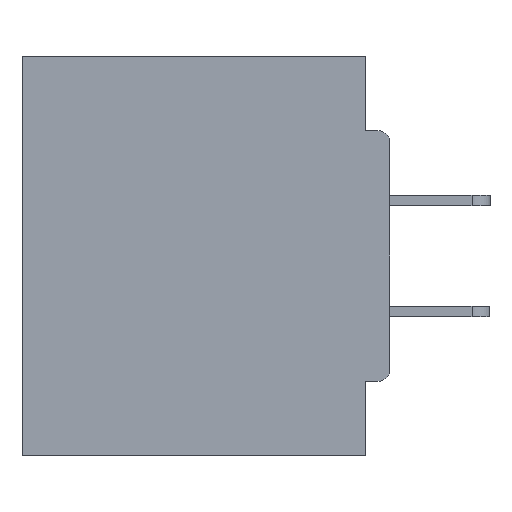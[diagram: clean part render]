
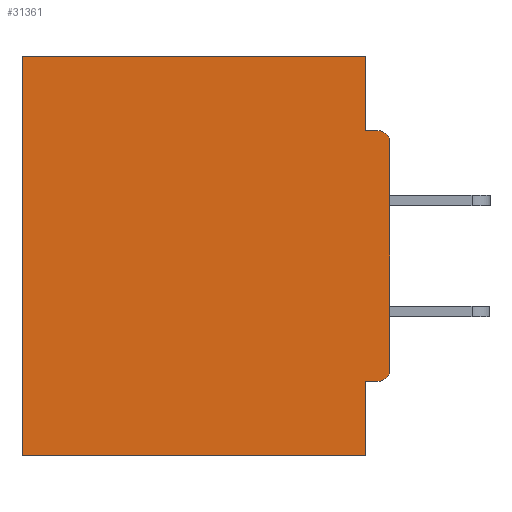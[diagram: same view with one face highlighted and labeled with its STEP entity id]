
A CAD part, left-side view. The second image highlights one B-rep face of the part: STEP entity #31361.
In plain terms, the highlighted planar face has unit normal (-1, 0, 0).
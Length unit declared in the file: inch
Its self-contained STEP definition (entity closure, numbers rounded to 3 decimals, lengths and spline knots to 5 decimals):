
#343 = VERTEX_POINT ( 'NONE', #32561 ) ;
#401 = VERTEX_POINT ( 'NONE', #16151 ) ;
#1222 = FACE_OUTER_BOUND ( 'NONE', #25110, .T. ) ;
#2314 = DIRECTION ( 'NONE',  ( 1., 0., 0. ) ) ;
#2408 = EDGE_CURVE ( 'NONE', #2842, #25228, #22369, .T. ) ;
#2842 = VERTEX_POINT ( 'NONE', #25498 ) ;
#3152 = DIRECTION ( 'NONE',  ( 0., 0., -1. ) ) ;
#3388 = ORIENTED_EDGE ( 'NONE', *, *, #12631, .T. ) ;
#3606 = CARTESIAN_POINT ( 'NONE',  ( 0.298, 0.015, -0.3915 ) ) ;
#3746 = ORIENTED_EDGE ( 'NONE', *, *, #28068, .F. ) ;
#3950 = VECTOR ( 'NONE', #13686, 39.37008 ) ;
#4068 = CARTESIAN_POINT ( 'NONE',  ( 0.298, 0., -0.0935 ) ) ;
#4237 = ORIENTED_EDGE ( 'NONE', *, *, #26782, .F. ) ;
#4886 = CARTESIAN_POINT ( 'NONE',  ( 0.298, 0., 0. ) ) ;
#5435 = DIRECTION ( 'NONE',  ( 0., 0., -1. ) ) ;
#5617 = DIRECTION ( 'NONE',  ( 0., 1., 0. ) ) ;
#6034 = DIRECTION ( 'NONE',  ( 0., 0., -1. ) ) ;
#6167 = CARTESIAN_POINT ( 'NONE',  ( 0.298, 0.46, 0. ) ) ;
#6882 = ORIENTED_EDGE ( 'NONE', *, *, #33731, .F. ) ;
#6929 = DIRECTION ( 'NONE',  ( 0., -1., 0. ) ) ;
#7746 = VERTEX_POINT ( 'NONE', #33199 ) ;
#8230 = VERTEX_POINT ( 'NONE', #6167 ) ;
#8473 = CARTESIAN_POINT ( 'NONE',  ( 0.298, 0., 0. ) ) ;
#8579 = CIRCLE ( 'NONE', #16238, 0.015 ) ;
#8806 = LINE ( 'NONE', #18816, #19209 ) ;
#9103 = AXIS2_PLACEMENT_3D ( 'NONE', #4886, #2314, #5435 ) ;
#9453 = EDGE_CURVE ( 'NONE', #2842, #8230, #15317, .T. ) ;
#9761 = LINE ( 'NONE', #23559, #26777 ) ;
#10464 = EDGE_CURVE ( 'NONE', #401, #15445, #8579, .T. ) ;
#10515 = CARTESIAN_POINT ( 'NONE',  ( 0.298, 0.031, -0.5 ) ) ;
#10682 = DIRECTION ( 'NONE',  ( 0., 0., -1. ) ) ;
#10738 = ORIENTED_EDGE ( 'NONE', *, *, #2408, .F. ) ;
#12617 = LINE ( 'NONE', #17740, #3950 ) ;
#12631 = EDGE_CURVE ( 'NONE', #7746, #22114, #14289, .T. ) ;
#12720 = PLANE ( 'NONE',  #9103 ) ;
#12870 = LINE ( 'NONE', #26684, #26172 ) ;
#13578 = DIRECTION ( 'NONE',  ( 0., 1., 0. ) ) ;
#13686 = DIRECTION ( 'NONE',  ( 0., 1., 0. ) ) ;
#14289 = CIRCLE ( 'NONE', #25843, 0.015 ) ;
#15317 = LINE ( 'NONE', #8473, #16559 ) ;
#15445 = VERTEX_POINT ( 'NONE', #31228 ) ;
#16151 = CARTESIAN_POINT ( 'NONE',  ( 0.298, 0., -0.1085 ) ) ;
#16238 = AXIS2_PLACEMENT_3D ( 'NONE', #16776, #30032, #25018 ) ;
#16546 = VERTEX_POINT ( 'NONE', #10515 ) ;
#16559 = VECTOR ( 'NONE', #13578, 39.37008 ) ;
#16776 = CARTESIAN_POINT ( 'NONE',  ( 0.298, 0.015, -0.1085 ) ) ;
#16864 = ORIENTED_EDGE ( 'NONE', *, *, #9453, .T. ) ;
#16934 = DIRECTION ( 'NONE',  ( -1., 0., 0. ) ) ;
#17408 = EDGE_CURVE ( 'NONE', #8230, #23121, #9761, .T. ) ;
#17567 = LINE ( 'NONE', #28535, #20471 ) ;
#17740 = CARTESIAN_POINT ( 'NONE',  ( 0.298, 0., -0.4065 ) ) ;
#18226 = EDGE_CURVE ( 'NONE', #401, #22114, #17567, .T. ) ;
#18816 = CARTESIAN_POINT ( 'NONE',  ( 0.298, 0., -0.5 ) ) ;
#19209 = VECTOR ( 'NONE', #5617, 39.37008 ) ;
#20423 = DIRECTION ( 'NONE',  ( 0., 0., -1. ) ) ;
#20471 = VECTOR ( 'NONE', #20978, 39.37008 ) ;
#20978 = DIRECTION ( 'NONE',  ( 0., 0., -1. ) ) ;
#22114 = VERTEX_POINT ( 'NONE', #25448 ) ;
#22369 = LINE ( 'NONE', #23090, #31997 ) ;
#23090 = CARTESIAN_POINT ( 'NONE',  ( 0.298, 0.031, -0.5 ) ) ;
#23121 = VERTEX_POINT ( 'NONE', #25894 ) ;
#23559 = CARTESIAN_POINT ( 'NONE',  ( 0.298, 0.46, 0. ) ) ;
#24185 = CARTESIAN_POINT ( 'NONE',  ( 0.298, 0.031, -0.0935 ) ) ;
#25018 = DIRECTION ( 'NONE',  ( 0., 0., -1. ) ) ;
#25062 = EDGE_CURVE ( 'NONE', #25228, #15445, #30523, .T. ) ;
#25110 = EDGE_LOOP ( 'NONE', ( #25555, #28040, #10738, #16864, #27936, #4237, #3746, #6882, #3388, #33179 ) ) ;
#25228 = VERTEX_POINT ( 'NONE', #24185 ) ;
#25448 = CARTESIAN_POINT ( 'NONE',  ( 0.298, 0., -0.3915 ) ) ;
#25498 = CARTESIAN_POINT ( 'NONE',  ( 0.298, 0.031, 0. ) ) ;
#25555 = ORIENTED_EDGE ( 'NONE', *, *, #10464, .T. ) ;
#25843 = AXIS2_PLACEMENT_3D ( 'NONE', #3606, #16934, #6034 ) ;
#25894 = CARTESIAN_POINT ( 'NONE',  ( 0.298, 0.46, -0.5 ) ) ;
#26172 = VECTOR ( 'NONE', #3152, 39.37008 ) ;
#26684 = CARTESIAN_POINT ( 'NONE',  ( 0.298, 0.031, -0.5 ) ) ;
#26777 = VECTOR ( 'NONE', #10682, 39.37008 ) ;
#26782 = EDGE_CURVE ( 'NONE', #16546, #23121, #8806, .T. ) ;
#27936 = ORIENTED_EDGE ( 'NONE', *, *, #17408, .T. ) ;
#28040 = ORIENTED_EDGE ( 'NONE', *, *, #25062, .F. ) ;
#28068 = EDGE_CURVE ( 'NONE', #343, #16546, #12870, .T. ) ;
#28535 = CARTESIAN_POINT ( 'NONE',  ( 0.298, 0., 0. ) ) ;
#29679 = VECTOR ( 'NONE', #6929, 39.37008 ) ;
#30032 = DIRECTION ( 'NONE',  ( -1., 0., 0. ) ) ;
#30523 = LINE ( 'NONE', #4068, #29679 ) ;
#31228 = CARTESIAN_POINT ( 'NONE',  ( 0.298, 0.015, -0.0935 ) ) ;
#31361 = ADVANCED_FACE ( 'NONE', ( #1222 ), #12720, .F. ) ;
#31997 = VECTOR ( 'NONE', #20423, 39.37008 ) ;
#32561 = CARTESIAN_POINT ( 'NONE',  ( 0.298, 0.031, -0.4065 ) ) ;
#33179 = ORIENTED_EDGE ( 'NONE', *, *, #18226, .F. ) ;
#33199 = CARTESIAN_POINT ( 'NONE',  ( 0.298, 0.015, -0.4065 ) ) ;
#33731 = EDGE_CURVE ( 'NONE', #7746, #343, #12617, .T. ) ;
